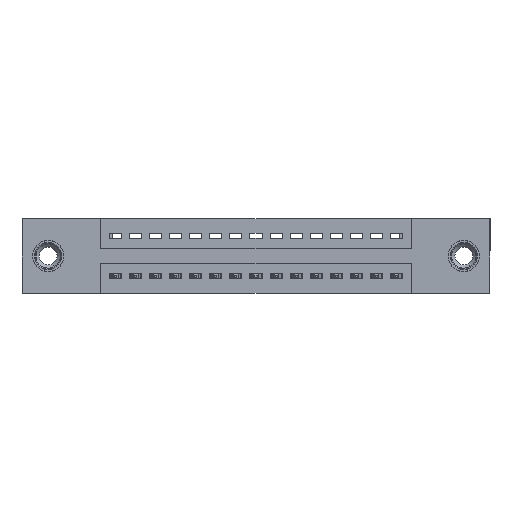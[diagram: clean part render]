
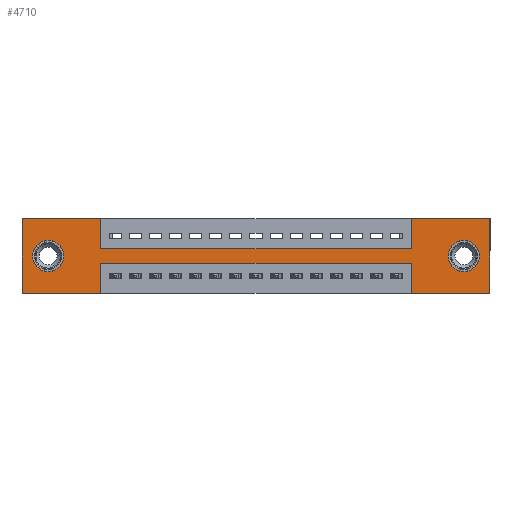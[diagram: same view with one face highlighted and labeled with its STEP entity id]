
A CAD part, front view. The second image highlights one B-rep face of the part: STEP entity #4710.
In plain terms, the highlighted planar face has unit normal (0, -1, 0).
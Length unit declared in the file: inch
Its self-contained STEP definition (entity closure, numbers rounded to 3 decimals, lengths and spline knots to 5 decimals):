
#186 = CIRCLE ( 'NONE', #16637, 0.078 ) ;
#323 = VECTOR ( 'NONE', #18293, 39.37008 ) ;
#646 = FACE_BOUND ( 'NONE', #16910, .T. ) ;
#761 = EDGE_CURVE ( 'NONE', #974, #12082, #186, .T. ) ;
#974 = VERTEX_POINT ( 'NONE', #9798 ) ;
#1007 = VERTEX_POINT ( 'NONE', #9253 ) ;
#1042 = CARTESIAN_POINT ( 'NONE',  ( 0., 0., -0.37 ) ) ;
#1429 = DIRECTION ( 'NONE',  ( 0., 1., 0. ) ) ;
#1433 = CARTESIAN_POINT ( 'NONE',  ( 0., 0., 0. ) ) ;
#1462 = ORIENTED_EDGE ( 'NONE', *, *, #16914, .F. ) ;
#1516 = EDGE_CURVE ( 'NONE', #19592, #1937, #3522, .T. ) ;
#1534 = CARTESIAN_POINT ( 'NONE',  ( 2.205, 0., -0.107 ) ) ;
#1707 = LINE ( 'NONE', #13729, #13361 ) ;
#1710 = CARTESIAN_POINT ( 'NONE',  ( 0.13, 0., -0.263 ) ) ;
#1766 = DIRECTION ( 'NONE',  ( 0., 0., 1. ) ) ;
#1891 = CARTESIAN_POINT ( 'NONE',  ( 1.9425, 0., -0.37 ) ) ;
#1937 = VERTEX_POINT ( 'NONE', #10858 ) ;
#1944 = VECTOR ( 'NONE', #3118, 39.37008 ) ;
#1965 = DIRECTION ( 'NONE',  ( 0., 0., 1. ) ) ;
#2214 = EDGE_CURVE ( 'NONE', #12938, #3547, #4214, .T. ) ;
#2357 = DIRECTION ( 'NONE',  ( 0., 0., -1. ) ) ;
#2586 = VERTEX_POINT ( 'NONE', #12066 ) ;
#2797 = ORIENTED_EDGE ( 'NONE', *, *, #17647, .F. ) ;
#2863 = CARTESIAN_POINT ( 'NONE',  ( 0.3925, 0., -0.15 ) ) ;
#2936 = VERTEX_POINT ( 'NONE', #1433 ) ;
#3118 = DIRECTION ( 'NONE',  ( 1., 0., 0. ) ) ;
#3197 = CARTESIAN_POINT ( 'NONE',  ( 0.3925, 0., -0.22 ) ) ;
#3212 = CARTESIAN_POINT ( 'NONE',  ( 0., 0., 0. ) ) ;
#3282 = VECTOR ( 'NONE', #7064, 39.37008 ) ;
#3391 = CARTESIAN_POINT ( 'NONE',  ( 1.9425, 0., -0.22 ) ) ;
#3437 = LINE ( 'NONE', #17034, #323 ) ;
#3487 = CARTESIAN_POINT ( 'NONE',  ( 1.9425, 0., 0. ) ) ;
#3522 = LINE ( 'NONE', #10996, #8289 ) ;
#3547 = VERTEX_POINT ( 'NONE', #6993 ) ;
#3587 = EDGE_CURVE ( 'NONE', #4597, #11883, #18009, .T. ) ;
#3857 = AXIS2_PLACEMENT_3D ( 'NONE', #6602, #18798, #5072 ) ;
#4127 = ORIENTED_EDGE ( 'NONE', *, *, #10450, .F. ) ;
#4147 = ORIENTED_EDGE ( 'NONE', *, *, #4383, .F. ) ;
#4214 = CIRCLE ( 'NONE', #7537, 0.078 ) ;
#4383 = EDGE_CURVE ( 'NONE', #1937, #8680, #19199, .T. ) ;
#4597 = VERTEX_POINT ( 'NONE', #5424 ) ;
#4644 = LINE ( 'NONE', #3212, #7251 ) ;
#4710 = ADVANCED_FACE ( 'NONE', ( #646, #15609, #19649 ), #5135, .T. ) ;
#5028 = DIRECTION ( 'NONE',  ( 0., 0., -1. ) ) ;
#5072 = DIRECTION ( 'NONE',  ( 0., 0., -1. ) ) ;
#5073 = CARTESIAN_POINT ( 'NONE',  ( 0., 0., -0.37 ) ) ;
#5135 = PLANE ( 'NONE',  #3857 ) ;
#5176 = CARTESIAN_POINT ( 'NONE',  ( 0.13, 0., -0.185 ) ) ;
#5270 = CIRCLE ( 'NONE', #6239, 0.078 ) ;
#5424 = CARTESIAN_POINT ( 'NONE',  ( 2.335, 0., -0.37 ) ) ;
#5972 = EDGE_LOOP ( 'NONE', ( #6625, #12153 ) ) ;
#6131 = ORIENTED_EDGE ( 'NONE', *, *, #8865, .T. ) ;
#6149 = DIRECTION ( 'NONE',  ( 1., 0., 0. ) ) ;
#6239 = AXIS2_PLACEMENT_3D ( 'NONE', #16167, #11606, #2357 ) ;
#6602 = CARTESIAN_POINT ( 'NONE',  ( 0., 0., -0.37 ) ) ;
#6625 = ORIENTED_EDGE ( 'NONE', *, *, #11843, .T. ) ;
#6840 = CARTESIAN_POINT ( 'NONE',  ( 1.9425, 0., 0. ) ) ;
#6993 = CARTESIAN_POINT ( 'NONE',  ( 0.13, 0., -0.107 ) ) ;
#7064 = DIRECTION ( 'NONE',  ( -1., 0., 0. ) ) ;
#7140 = EDGE_CURVE ( 'NONE', #2936, #7945, #4644, .T. ) ;
#7236 = LINE ( 'NONE', #3487, #14592 ) ;
#7251 = VECTOR ( 'NONE', #13844, 39.37008 ) ;
#7291 = CARTESIAN_POINT ( 'NONE',  ( 1.9425, 0., -0.37 ) ) ;
#7320 = CIRCLE ( 'NONE', #14229, 0.078 ) ;
#7527 = LINE ( 'NONE', #3197, #15099 ) ;
#7537 = AXIS2_PLACEMENT_3D ( 'NONE', #5176, #15658, #1965 ) ;
#7786 = DIRECTION ( 'NONE',  ( -1., 0., 0. ) ) ;
#7945 = VERTEX_POINT ( 'NONE', #14952 ) ;
#8289 = VECTOR ( 'NONE', #12523, 39.37008 ) ;
#8680 = VERTEX_POINT ( 'NONE', #5073 ) ;
#8865 = EDGE_CURVE ( 'NONE', #12082, #974, #5270, .T. ) ;
#9228 = EDGE_CURVE ( 'NONE', #2586, #13188, #7236, .T. ) ;
#9252 = VECTOR ( 'NONE', #16881, 39.37008 ) ;
#9253 = CARTESIAN_POINT ( 'NONE',  ( 2.335, 0., 0. ) ) ;
#9313 = VECTOR ( 'NONE', #1766, 39.37008 ) ;
#9444 = CARTESIAN_POINT ( 'NONE',  ( 0.3925, 0., -0.15 ) ) ;
#9563 = ORIENTED_EDGE ( 'NONE', *, *, #3587, .F. ) ;
#9798 = CARTESIAN_POINT ( 'NONE',  ( 2.205, 0., -0.263 ) ) ;
#9868 = ORIENTED_EDGE ( 'NONE', *, *, #15822, .F. ) ;
#10133 = DIRECTION ( 'NONE',  ( 0., 1., 0. ) ) ;
#10450 = EDGE_CURVE ( 'NONE', #8680, #2936, #15203, .T. ) ;
#10544 = LINE ( 'NONE', #9444, #1944 ) ;
#10730 = ORIENTED_EDGE ( 'NONE', *, *, #7140, .F. ) ;
#10858 = CARTESIAN_POINT ( 'NONE',  ( 0.3925, 0., -0.37 ) ) ;
#10949 = ORIENTED_EDGE ( 'NONE', *, *, #15275, .F. ) ;
#10996 = CARTESIAN_POINT ( 'NONE',  ( 0.3925, 0., -0.37 ) ) ;
#11606 = DIRECTION ( 'NONE',  ( 0., 1., 0. ) ) ;
#11831 = ORIENTED_EDGE ( 'NONE', *, *, #9228, .F. ) ;
#11843 = EDGE_CURVE ( 'NONE', #3547, #12938, #7320, .T. ) ;
#11883 = VERTEX_POINT ( 'NONE', #7291 ) ;
#11925 = DIRECTION ( 'NONE',  ( 0., 0., 1. ) ) ;
#12066 = CARTESIAN_POINT ( 'NONE',  ( 1.9425, 0., -0.15 ) ) ;
#12082 = VERTEX_POINT ( 'NONE', #1534 ) ;
#12136 = VERTEX_POINT ( 'NONE', #2863 ) ;
#12153 = ORIENTED_EDGE ( 'NONE', *, *, #2214, .T. ) ;
#12523 = DIRECTION ( 'NONE',  ( 0., 0., -1. ) ) ;
#12938 = VERTEX_POINT ( 'NONE', #1710 ) ;
#13031 = DIRECTION ( 'NONE',  ( 0., 0., 1. ) ) ;
#13161 = ORIENTED_EDGE ( 'NONE', *, *, #761, .T. ) ;
#13173 = DIRECTION ( 'NONE',  ( 0., 0., -1. ) ) ;
#13188 = VERTEX_POINT ( 'NONE', #6840 ) ;
#13361 = VECTOR ( 'NONE', #6149, 39.37008 ) ;
#13729 = CARTESIAN_POINT ( 'NONE',  ( 0., 0., 0. ) ) ;
#13844 = DIRECTION ( 'NONE',  ( 1., 0., 0. ) ) ;
#14229 = AXIS2_PLACEMENT_3D ( 'NONE', #16557, #1429, #11925 ) ;
#14333 = ORIENTED_EDGE ( 'NONE', *, *, #14898, .F. ) ;
#14592 = VECTOR ( 'NONE', #18421, 39.37008 ) ;
#14898 = EDGE_CURVE ( 'NONE', #1007, #4597, #17644, .T. ) ;
#14952 = CARTESIAN_POINT ( 'NONE',  ( 0.3925, 0., 0. ) ) ;
#15004 = LINE ( 'NONE', #1891, #9313 ) ;
#15099 = VECTOR ( 'NONE', #7786, 39.37008 ) ;
#15203 = LINE ( 'NONE', #17538, #17786 ) ;
#15261 = VERTEX_POINT ( 'NONE', #3391 ) ;
#15275 = EDGE_CURVE ( 'NONE', #12136, #2586, #10544, .T. ) ;
#15520 = EDGE_LOOP ( 'NONE', ( #18004, #1462, #9868, #9563, #14333, #17714, #11831, #10949, #2797, #10730, #4127, #4147 ) ) ;
#15609 = FACE_BOUND ( 'NONE', #5972, .T. ) ;
#15658 = DIRECTION ( 'NONE',  ( 0., 1., 0. ) ) ;
#15822 = EDGE_CURVE ( 'NONE', #11883, #15261, #15004, .T. ) ;
#16167 = CARTESIAN_POINT ( 'NONE',  ( 2.205, 0., -0.185 ) ) ;
#16557 = CARTESIAN_POINT ( 'NONE',  ( 0.13, 0., -0.185 ) ) ;
#16637 = AXIS2_PLACEMENT_3D ( 'NONE', #17665, #10133, #13173 ) ;
#16881 = DIRECTION ( 'NONE',  ( -1., 0., 0. ) ) ;
#16910 = EDGE_LOOP ( 'NONE', ( #6131, #13161 ) ) ;
#16914 = EDGE_CURVE ( 'NONE', #15261, #19592, #7527, .T. ) ;
#17034 = CARTESIAN_POINT ( 'NONE',  ( 0.3925, 0., 0. ) ) ;
#17282 = CARTESIAN_POINT ( 'NONE',  ( 2.335, 0., 0. ) ) ;
#17538 = CARTESIAN_POINT ( 'NONE',  ( 0., 0., 0. ) ) ;
#17644 = LINE ( 'NONE', #17282, #18606 ) ;
#17647 = EDGE_CURVE ( 'NONE', #7945, #12136, #3437, .T. ) ;
#17665 = CARTESIAN_POINT ( 'NONE',  ( 2.205, 0., -0.185 ) ) ;
#17714 = ORIENTED_EDGE ( 'NONE', *, *, #18763, .F. ) ;
#17778 = CARTESIAN_POINT ( 'NONE',  ( 0., 0., -0.37 ) ) ;
#17786 = VECTOR ( 'NONE', #13031, 39.37008 ) ;
#18004 = ORIENTED_EDGE ( 'NONE', *, *, #1516, .F. ) ;
#18009 = LINE ( 'NONE', #1042, #9252 ) ;
#18293 = DIRECTION ( 'NONE',  ( 0., 0., -1. ) ) ;
#18421 = DIRECTION ( 'NONE',  ( 0., 0., 1. ) ) ;
#18606 = VECTOR ( 'NONE', #5028, 39.37008 ) ;
#18763 = EDGE_CURVE ( 'NONE', #13188, #1007, #1707, .T. ) ;
#18798 = DIRECTION ( 'NONE',  ( 0., -1., 0. ) ) ;
#19001 = CARTESIAN_POINT ( 'NONE',  ( 0.3925, 0., -0.22 ) ) ;
#19199 = LINE ( 'NONE', #17778, #3282 ) ;
#19592 = VERTEX_POINT ( 'NONE', #19001 ) ;
#19649 = FACE_OUTER_BOUND ( 'NONE', #15520, .T. ) ;
